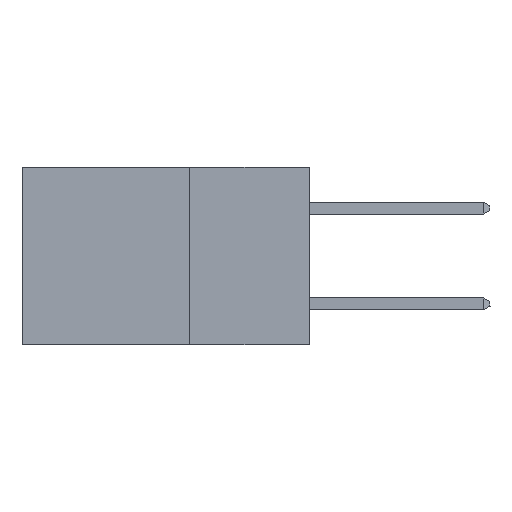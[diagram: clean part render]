
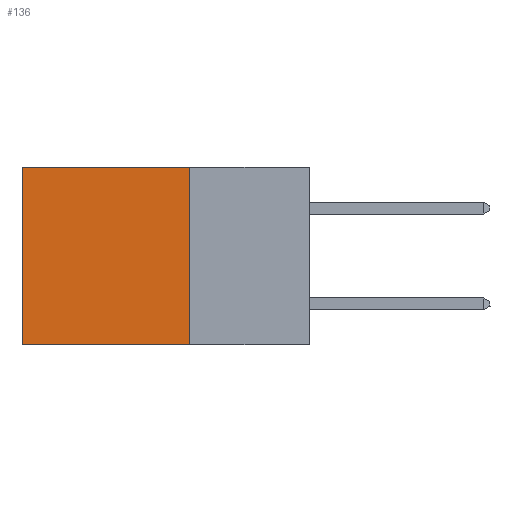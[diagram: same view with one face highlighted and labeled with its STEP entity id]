
A CAD part, left-side view. The second image highlights one B-rep face of the part: STEP entity #136.
In plain terms, the highlighted planar face has unit normal (-1, 0, 0).
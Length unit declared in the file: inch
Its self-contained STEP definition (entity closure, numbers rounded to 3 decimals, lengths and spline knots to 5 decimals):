
#136 = ADVANCED_FACE ( 'NONE', ( #9094 ), #11656, .F. ) ;
#4275 = LINE ( 'NONE', #5554, #28267 ) ;
#4569 = VERTEX_POINT ( 'NONE', #18333 ) ;
#4944 = EDGE_CURVE ( 'NONE', #24106, #24716, #4275, .T. ) ;
#5481 = DIRECTION ( 'NONE',  ( 0., 1., 0. ) ) ;
#5554 = CARTESIAN_POINT ( 'NONE',  ( 0.2875, 0.25, -0.37 ) ) ;
#5924 = CARTESIAN_POINT ( 'NONE',  ( 0.2875, 0.6, 0. ) ) ;
#7951 = DIRECTION ( 'NONE',  ( 0., 1., 0. ) ) ;
#8261 = EDGE_CURVE ( 'NONE', #18153, #4569, #28491, .T. ) ;
#8573 = DIRECTION ( 'NONE',  ( 0., 0., -1. ) ) ;
#8791 = CARTESIAN_POINT ( 'NONE',  ( 0.2875, 0.25, 0. ) ) ;
#9050 = ORIENTED_EDGE ( 'NONE', *, *, #10675, .T. ) ;
#9094 = FACE_OUTER_BOUND ( 'NONE', #25119, .T. ) ;
#10372 = CARTESIAN_POINT ( 'NONE',  ( 0.2875, 0.25, 0. ) ) ;
#10675 = EDGE_CURVE ( 'NONE', #4569, #24716, #23822, .T. ) ;
#11656 = PLANE ( 'NONE',  #27165 ) ;
#11730 = LINE ( 'NONE', #8791, #12055 ) ;
#11835 = VECTOR ( 'NONE', #20358, 39.37008 ) ;
#11939 = VECTOR ( 'NONE', #5481, 39.37008 ) ;
#12055 = VECTOR ( 'NONE', #8573, 39.37008 ) ;
#12101 = ORIENTED_EDGE ( 'NONE', *, *, #4944, .F. ) ;
#12393 = ORIENTED_EDGE ( 'NONE', *, *, #8261, .T. ) ;
#14193 = CARTESIAN_POINT ( 'NONE',  ( 0.2875, 0.25, 0. ) ) ;
#16423 = CARTESIAN_POINT ( 'NONE',  ( 0.2875, 0.25, 0. ) ) ;
#18153 = VERTEX_POINT ( 'NONE', #14193 ) ;
#18333 = CARTESIAN_POINT ( 'NONE',  ( 0.2875, 0.6, 0. ) ) ;
#19529 = CARTESIAN_POINT ( 'NONE',  ( 0.2875, 0.6, -0.37 ) ) ;
#19693 = ORIENTED_EDGE ( 'NONE', *, *, #24221, .F. ) ;
#20358 = DIRECTION ( 'NONE',  ( 0., 0., -1. ) ) ;
#23822 = LINE ( 'NONE', #5924, #11835 ) ;
#24106 = VERTEX_POINT ( 'NONE', #24711 ) ;
#24221 = EDGE_CURVE ( 'NONE', #18153, #24106, #11730, .T. ) ;
#24711 = CARTESIAN_POINT ( 'NONE',  ( 0.2875, 0.25, -0.37 ) ) ;
#24716 = VERTEX_POINT ( 'NONE', #19529 ) ;
#25119 = EDGE_LOOP ( 'NONE', ( #9050, #12101, #19693, #12393 ) ) ;
#26853 = DIRECTION ( 'NONE',  ( 0., 0., -1. ) ) ;
#27165 = AXIS2_PLACEMENT_3D ( 'NONE', #16423, #30948, #26853 ) ;
#28267 = VECTOR ( 'NONE', #7951, 39.37008 ) ;
#28491 = LINE ( 'NONE', #10372, #11939 ) ;
#30948 = DIRECTION ( 'NONE',  ( 1., 0., 0. ) ) ;
